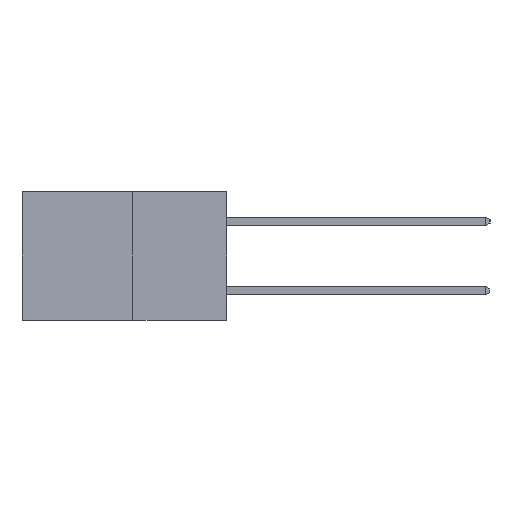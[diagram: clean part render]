
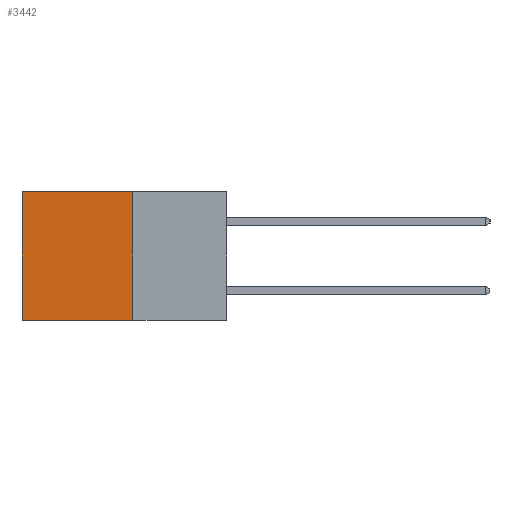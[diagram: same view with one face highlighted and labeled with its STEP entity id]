
A CAD part, left-side view. The second image highlights one B-rep face of the part: STEP entity #3442.
In plain terms, the highlighted planar face has unit normal (-1, 0, 0).
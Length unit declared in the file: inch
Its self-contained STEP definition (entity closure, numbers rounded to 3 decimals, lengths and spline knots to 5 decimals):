
#1429 = CARTESIAN_POINT ( 'NONE',  ( 0.277, 0.59, 0. ) ) ;
#2035 = ORIENTED_EDGE ( 'NONE', *, *, #17983, .F. ) ;
#2232 = CARTESIAN_POINT ( 'NONE',  ( 0.277, 0.27, -0.37 ) ) ;
#2331 = CARTESIAN_POINT ( 'NONE',  ( 0.277, 0.59, -0.37 ) ) ;
#2677 = LINE ( 'NONE', #10721, #10611 ) ;
#3442 = ADVANCED_FACE ( 'NONE', ( #14617 ), #16053, .F. ) ;
#4179 = LINE ( 'NONE', #7941, #8901 ) ;
#6282 = ORIENTED_EDGE ( 'NONE', *, *, #18798, .T. ) ;
#6745 = DIRECTION ( 'NONE',  ( 0., 1., 0. ) ) ;
#7682 = EDGE_LOOP ( 'NONE', ( #8507, #9490, #2035, #6282 ) ) ;
#7941 = CARTESIAN_POINT ( 'NONE',  ( 0.277, 0.27, -0.37 ) ) ;
#8507 = ORIENTED_EDGE ( 'NONE', *, *, #11799, .T. ) ;
#8751 = CARTESIAN_POINT ( 'NONE',  ( 0.277, 0.27, 0. ) ) ;
#8901 = VECTOR ( 'NONE', #17286, 39.37008 ) ;
#9490 = ORIENTED_EDGE ( 'NONE', *, *, #19144, .F. ) ;
#10611 = VECTOR ( 'NONE', #12285, 39.37008 ) ;
#10721 = CARTESIAN_POINT ( 'NONE',  ( 0.277, 0.27, -0.37 ) ) ;
#10777 = AXIS2_PLACEMENT_3D ( 'NONE', #18543, #18437, #18364 ) ;
#10781 = VERTEX_POINT ( 'NONE', #2232 ) ;
#11799 = EDGE_CURVE ( 'NONE', #12766, #18960, #13517, .T. ) ;
#11994 = CARTESIAN_POINT ( 'NONE',  ( 0.277, 0.59, -0.37 ) ) ;
#12285 = DIRECTION ( 'NONE',  ( 0., 1., 0. ) ) ;
#12766 = VERTEX_POINT ( 'NONE', #1429 ) ;
#13000 = CARTESIAN_POINT ( 'NONE',  ( 0.277, 0.27, 0. ) ) ;
#13517 = LINE ( 'NONE', #11994, #14029 ) ;
#14029 = VECTOR ( 'NONE', #16716, 39.37008 ) ;
#14392 = VERTEX_POINT ( 'NONE', #8751 ) ;
#14617 = FACE_OUTER_BOUND ( 'NONE', #7682, .T. ) ;
#16053 = PLANE ( 'NONE',  #10777 ) ;
#16716 = DIRECTION ( 'NONE',  ( 0., 0., -1. ) ) ;
#17286 = DIRECTION ( 'NONE',  ( 0., 0., -1. ) ) ;
#17444 = VECTOR ( 'NONE', #6745, 39.37008 ) ;
#17910 = LINE ( 'NONE', #13000, #17444 ) ;
#17983 = EDGE_CURVE ( 'NONE', #14392, #10781, #4179, .T. ) ;
#18364 = DIRECTION ( 'NONE',  ( 0., 0., -1. ) ) ;
#18437 = DIRECTION ( 'NONE',  ( 1., 0., 0. ) ) ;
#18543 = CARTESIAN_POINT ( 'NONE',  ( 0.277, 0.27, -0.37 ) ) ;
#18798 = EDGE_CURVE ( 'NONE', #14392, #12766, #17910, .T. ) ;
#18960 = VERTEX_POINT ( 'NONE', #2331 ) ;
#19144 = EDGE_CURVE ( 'NONE', #10781, #18960, #2677, .T. ) ;
